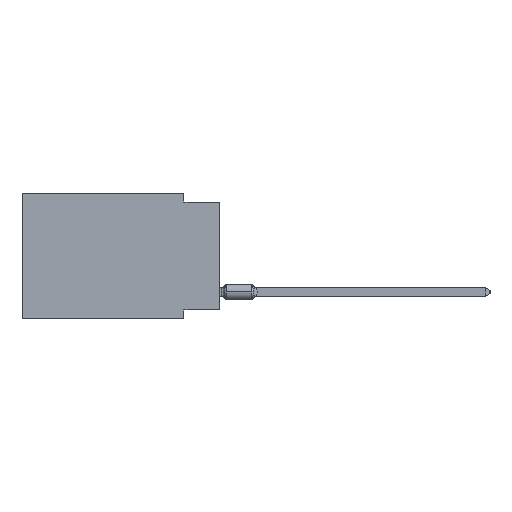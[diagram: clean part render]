
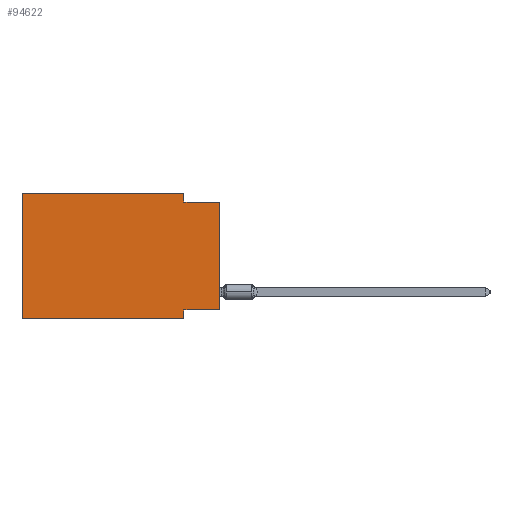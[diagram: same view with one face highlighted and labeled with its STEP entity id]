
A CAD part, left-side view. The second image highlights one B-rep face of the part: STEP entity #94622.
In plain terms, the highlighted planar face has unit normal (-1, 0, 0).
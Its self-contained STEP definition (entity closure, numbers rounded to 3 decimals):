
#789 = VERTEX_POINT ( 'NONE', #21065 ) ;
#818 = CARTESIAN_POINT ( 'NONE',  ( 0., 13.97, 0. ) ) ;
#922 = CARTESIAN_POINT ( 'NONE',  ( 0., 2.54, 0. ) ) ;
#1421 = DIRECTION ( 'NONE',  ( 0., 0., -1. ) ) ;
#3485 = CARTESIAN_POINT ( 'NONE',  ( 0., 13.97, 0. ) ) ;
#5399 = CARTESIAN_POINT ( 'NONE',  ( 0., 2.54, -0.635 ) ) ;
#8071 = VECTOR ( 'NONE', #95808, 1000. ) ;
#8380 = VECTOR ( 'NONE', #97015, 1000. ) ;
#8479 = DIRECTION ( 'NONE',  ( 0., 0., -1. ) ) ;
#10176 = LINE ( 'NONE', #25528, #78219 ) ;
#10724 = VERTEX_POINT ( 'NONE', #24088 ) ;
#12881 = LINE ( 'NONE', #34910, #58141 ) ;
#14067 = ORIENTED_EDGE ( 'NONE', *, *, #67562, .F. ) ;
#19332 = LINE ( 'NONE', #41386, #49318 ) ;
#19502 = LINE ( 'NONE', #65101, #53485 ) ;
#19539 = DIRECTION ( 'NONE',  ( 0., -1., 0. ) ) ;
#21065 = CARTESIAN_POINT ( 'NONE',  ( 0., 2.54, -8.255 ) ) ;
#21107 = CARTESIAN_POINT ( 'NONE',  ( 0., 2.54, 0. ) ) ;
#21877 = VERTEX_POINT ( 'NONE', #91199 ) ;
#22907 = ORIENTED_EDGE ( 'NONE', *, *, #96385, .F. ) ;
#24088 = CARTESIAN_POINT ( 'NONE',  ( 0., 0., -8.255 ) ) ;
#24709 = EDGE_CURVE ( 'NONE', #77890, #40993, #70497, .T. ) ;
#25528 = CARTESIAN_POINT ( 'NONE',  ( 0., 2.54, -8.89 ) ) ;
#25818 = DIRECTION ( 'NONE',  ( 1., 0., 0. ) ) ;
#26451 = LINE ( 'NONE', #35649, #8380 ) ;
#30313 = EDGE_CURVE ( 'NONE', #99215, #76712, #19502, .T. ) ;
#30518 = CARTESIAN_POINT ( 'NONE',  ( 0., 13.97, 0. ) ) ;
#33198 = EDGE_CURVE ( 'NONE', #789, #21877, #10176, .T. ) ;
#34910 = CARTESIAN_POINT ( 'NONE',  ( 0., 0., -0.635 ) ) ;
#35649 = CARTESIAN_POINT ( 'NONE',  ( 0., 0., -8.255 ) ) ;
#38444 = VECTOR ( 'NONE', #44858, 1000. ) ;
#39494 = ORIENTED_EDGE ( 'NONE', *, *, #81847, .T. ) ;
#40254 = ORIENTED_EDGE ( 'NONE', *, *, #24709, .F. ) ;
#40993 = VERTEX_POINT ( 'NONE', #5399 ) ;
#41386 = CARTESIAN_POINT ( 'NONE',  ( 0., 13.97, -8.89 ) ) ;
#44858 = DIRECTION ( 'NONE',  ( 0., -1., 0. ) ) ;
#46384 = LINE ( 'NONE', #30518, #38444 ) ;
#49318 = VECTOR ( 'NONE', #57741, 1000. ) ;
#50270 = LINE ( 'NONE', #65138, #8071 ) ;
#52861 = CARTESIAN_POINT ( 'NONE',  ( 0., 0., -0.635 ) ) ;
#53485 = VECTOR ( 'NONE', #72281, 1000. ) ;
#54089 = VERTEX_POINT ( 'NONE', #52861 ) ;
#56498 = ORIENTED_EDGE ( 'NONE', *, *, #73725, .F. ) ;
#57741 = DIRECTION ( 'NONE',  ( 0., -1., 0. ) ) ;
#57992 = EDGE_CURVE ( 'NONE', #99215, #21877, #19332, .T. ) ;
#58141 = VECTOR ( 'NONE', #19539, 1000. ) ;
#62943 = ORIENTED_EDGE ( 'NONE', *, *, #30313, .F. ) ;
#63502 = EDGE_LOOP ( 'NONE', ( #39494, #22907, #40254, #56498, #62943, #100388, #100309, #14067 ) ) ;
#64730 = PLANE ( 'NONE',  #80768 ) ;
#65101 = CARTESIAN_POINT ( 'NONE',  ( 0., 13.97, 0. ) ) ;
#65138 = CARTESIAN_POINT ( 'NONE',  ( 0., 0., 0. ) ) ;
#67562 = EDGE_CURVE ( 'NONE', #10724, #789, #26451, .T. ) ;
#68654 = VECTOR ( 'NONE', #1421, 1000. ) ;
#70497 = LINE ( 'NONE', #922, #68654 ) ;
#72281 = DIRECTION ( 'NONE',  ( 0., 0., 1. ) ) ;
#73725 = EDGE_CURVE ( 'NONE', #76712, #77890, #46384, .T. ) ;
#76712 = VERTEX_POINT ( 'NONE', #3485 ) ;
#77890 = VERTEX_POINT ( 'NONE', #21107 ) ;
#78219 = VECTOR ( 'NONE', #79759, 1000. ) ;
#79759 = DIRECTION ( 'NONE',  ( 0., 0., -1. ) ) ;
#80768 = AXIS2_PLACEMENT_3D ( 'NONE', #818, #25818, #8479 ) ;
#81847 = EDGE_CURVE ( 'NONE', #10724, #54089, #50270, .T. ) ;
#87219 = FACE_OUTER_BOUND ( 'NONE', #63502, .T. ) ;
#88431 = CARTESIAN_POINT ( 'NONE',  ( 0., 13.97, -8.89 ) ) ;
#91199 = CARTESIAN_POINT ( 'NONE',  ( 0., 2.54, -8.89 ) ) ;
#94622 = ADVANCED_FACE ( 'NONE', ( #87219 ), #64730, .F. ) ;
#95808 = DIRECTION ( 'NONE',  ( 0., 0., 1. ) ) ;
#96385 = EDGE_CURVE ( 'NONE', #40993, #54089, #12881, .T. ) ;
#97015 = DIRECTION ( 'NONE',  ( 0., 1., 0. ) ) ;
#99215 = VERTEX_POINT ( 'NONE', #88431 ) ;
#100309 = ORIENTED_EDGE ( 'NONE', *, *, #33198, .F. ) ;
#100388 = ORIENTED_EDGE ( 'NONE', *, *, #57992, .T. ) ;
